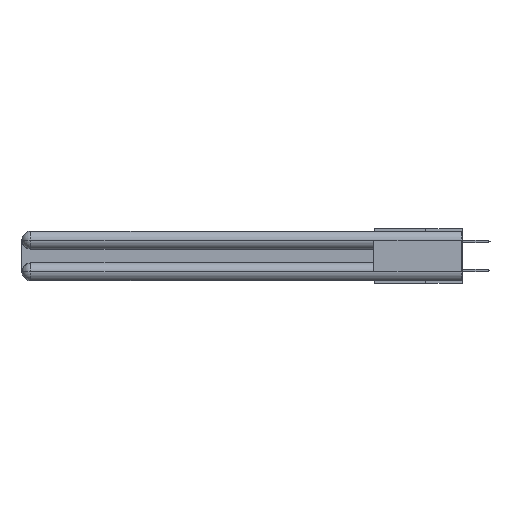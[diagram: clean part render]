
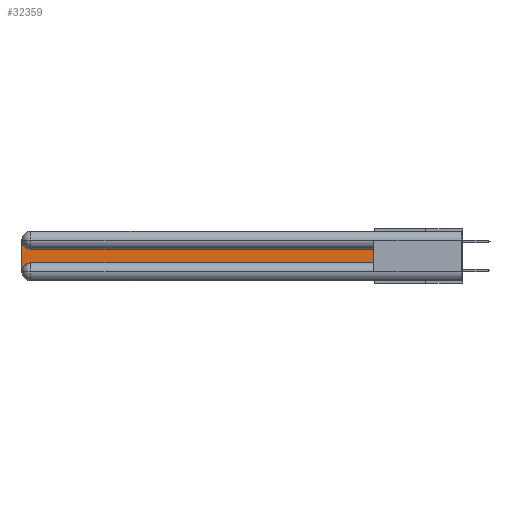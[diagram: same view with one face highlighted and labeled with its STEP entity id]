
A CAD part, left-side view. The second image highlights one B-rep face of the part: STEP entity #32359.
In plain terms, the highlighted planar face has unit normal (-1, 0, 0).
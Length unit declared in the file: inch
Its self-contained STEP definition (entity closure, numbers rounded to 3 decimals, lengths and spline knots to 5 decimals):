
#102 = CARTESIAN_POINT ( 'NONE',  ( 0.075, 3., -0.2175 ) ) ;
#1104 = CARTESIAN_POINT ( 'NONE',  ( 0.075, 0.6, -0.2175 ) ) ;
#1983 = LINE ( 'NONE', #30329, #8166 ) ;
#2002 = DIRECTION ( 'NONE',  ( 0., -1., 0. ) ) ;
#2145 = ORIENTED_EDGE ( 'NONE', *, *, #22824, .T. ) ;
#2388 = VERTEX_POINT ( 'NONE', #18933 ) ;
#3152 = VERTEX_POINT ( 'NONE', #22474 ) ;
#4083 = DIRECTION ( 'NONE',  ( 0., 0., -1. ) ) ;
#4181 = ORIENTED_EDGE ( 'NONE', *, *, #5053, .T. ) ;
#5053 = EDGE_CURVE ( 'NONE', #10008, #16044, #30817, .T. ) ;
#5149 = EDGE_CURVE ( 'NONE', #2388, #28866, #25132, .T. ) ;
#5551 = DIRECTION ( 'NONE',  ( 1., 0., 0. ) ) ;
#6724 = CARTESIAN_POINT ( 'NONE',  ( 0.075, 0.6, -0.2175 ) ) ;
#8012 = VECTOR ( 'NONE', #15437, 39.37008 ) ;
#8166 = VECTOR ( 'NONE', #22562, 39.37008 ) ;
#9269 = DIRECTION ( 'NONE',  ( 1., 0., 0. ) ) ;
#9517 = EDGE_CURVE ( 'NONE', #3152, #2388, #11833, .T. ) ;
#9576 = ORIENTED_EDGE ( 'NONE', *, *, #16982, .T. ) ;
#10008 = VERTEX_POINT ( 'NONE', #11155 ) ;
#10102 = AXIS2_PLACEMENT_3D ( 'NONE', #19758, #9269, #4083 ) ;
#11155 = CARTESIAN_POINT ( 'NONE',  ( 0.075, 2.94, -0.1225 ) ) ;
#11640 = AXIS2_PLACEMENT_3D ( 'NONE', #19020, #5551, #13840 ) ;
#11833 = LINE ( 'NONE', #6724, #34039 ) ;
#12421 = CARTESIAN_POINT ( 'NONE',  ( 0.075, 0.6, -0.1225 ) ) ;
#13840 = DIRECTION ( 'NONE',  ( 0., 0., -1. ) ) ;
#14686 = AXIS2_PLACEMENT_3D ( 'NONE', #26385, #29338, #21091 ) ;
#15437 = DIRECTION ( 'NONE',  ( 0., 0., -1. ) ) ;
#16044 = VERTEX_POINT ( 'NONE', #16438 ) ;
#16409 = PLANE ( 'NONE',  #11640 ) ;
#16438 = CARTESIAN_POINT ( 'NONE',  ( 0.075, 3., -0.0625 ) ) ;
#16982 = EDGE_CURVE ( 'NONE', #16044, #22153, #22412, .T. ) ;
#17877 = FACE_OUTER_BOUND ( 'NONE', #33706, .T. ) ;
#17988 = ORIENTED_EDGE ( 'NONE', *, *, #9517, .T. ) ;
#18155 = VECTOR ( 'NONE', #20531, 39.37008 ) ;
#18933 = CARTESIAN_POINT ( 'NONE',  ( 0.075, 0.6, -0.2175 ) ) ;
#19020 = CARTESIAN_POINT ( 'NONE',  ( 0.075, 3., -0.1225 ) ) ;
#19758 = CARTESIAN_POINT ( 'NONE',  ( 0.075, 2.94, -0.0625 ) ) ;
#20219 = ORIENTED_EDGE ( 'NONE', *, *, #5149, .T. ) ;
#20531 = DIRECTION ( 'NONE',  ( 0., 0., 1. ) ) ;
#21091 = DIRECTION ( 'NONE',  ( 0., 0., -1. ) ) ;
#22153 = VERTEX_POINT ( 'NONE', #29810 ) ;
#22412 = LINE ( 'NONE', #102, #8012 ) ;
#22474 = CARTESIAN_POINT ( 'NONE',  ( 0.075, 2.94, -0.2175 ) ) ;
#22562 = DIRECTION ( 'NONE',  ( 0., 1., 0. ) ) ;
#22824 = EDGE_CURVE ( 'NONE', #28866, #10008, #1983, .T. ) ;
#25132 = LINE ( 'NONE', #1104, #18155 ) ;
#26385 = CARTESIAN_POINT ( 'NONE',  ( 0.075, 2.94, -0.2775 ) ) ;
#26662 = CIRCLE ( 'NONE', #14686, 0.06 ) ;
#28213 = EDGE_CURVE ( 'NONE', #22153, #3152, #26662, .T. ) ;
#28866 = VERTEX_POINT ( 'NONE', #12421 ) ;
#29338 = DIRECTION ( 'NONE',  ( 1., 0., 0. ) ) ;
#29810 = CARTESIAN_POINT ( 'NONE',  ( 0.075, 3., -0.2775 ) ) ;
#30329 = CARTESIAN_POINT ( 'NONE',  ( 0.075, 0.6, -0.1225 ) ) ;
#30817 = CIRCLE ( 'NONE', #10102, 0.06 ) ;
#32359 = ADVANCED_FACE ( 'NONE', ( #17877 ), #16409, .F. ) ;
#32500 = ORIENTED_EDGE ( 'NONE', *, *, #28213, .T. ) ;
#33706 = EDGE_LOOP ( 'NONE', ( #2145, #4181, #9576, #32500, #17988, #20219 ) ) ;
#34039 = VECTOR ( 'NONE', #2002, 39.37008 ) ;
